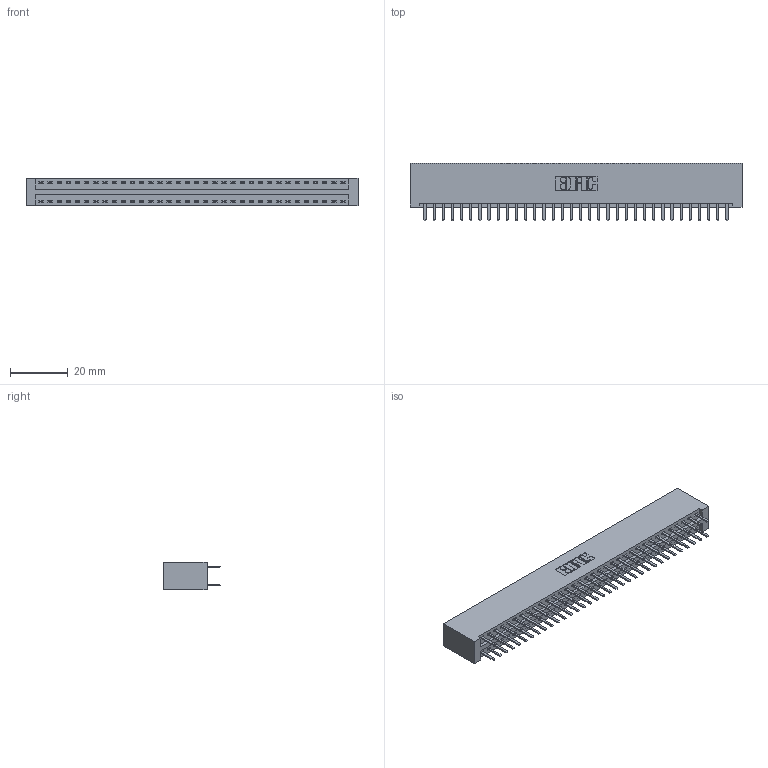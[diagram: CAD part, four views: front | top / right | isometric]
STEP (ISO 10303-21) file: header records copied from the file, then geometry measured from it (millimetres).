
FILE_DESCRIPTION (( 'STEP AP203' ), '1' );
FILE_NAME ('346-068-520-201.STEP', '2018-08-28T12:04:36', ( '' ), ( '' ), 'SwSTEP 2.0', 'SolidWorks 2016', '' );
FILE_SCHEMA (( 'CONFIG_CONTROL_DESIGN' ));
Length unit declared in the file: inch
Products named in the file (3): 346 Part_No Mounting Lugs; 345-292-001_345-293-120; 346-068-520-201
Assembly tree (69 placements, depth 2):
  346-068-520-201
    346 Part_No Mounting Lugs
    345-292-001_345-293-120  x68
Bounding box: 115.19 x 20.02 x 9.4 mm (x, y, z)
Volume: 11713.6 mm3; surface area: 16068.6 mm2
Topology: 69 solids, 69 shells, 3922 faces, 11389 edges, 7410 vertices
Faces by surface type: plane 2588, cylinder 1334
Entity records: 23103 total; most frequent: CARTESIAN_POINT 3828, ORIENTED_EDGE 3750, DIRECTION 3407, EDGE_CURVE 1875, LINE 1611, VECTOR 1611, VERTEX_POINT 1246, AXIS2_PLACEMENT_3D 898
